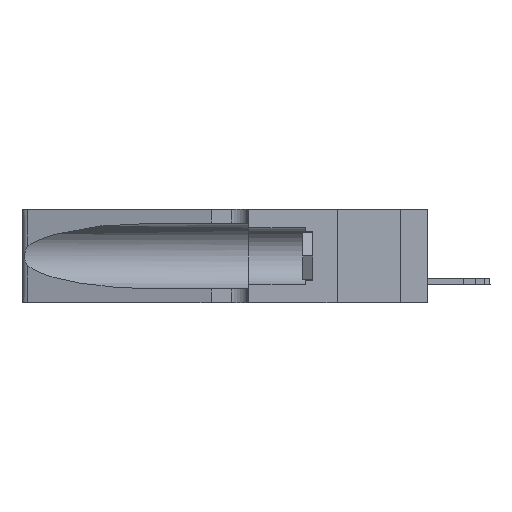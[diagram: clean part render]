
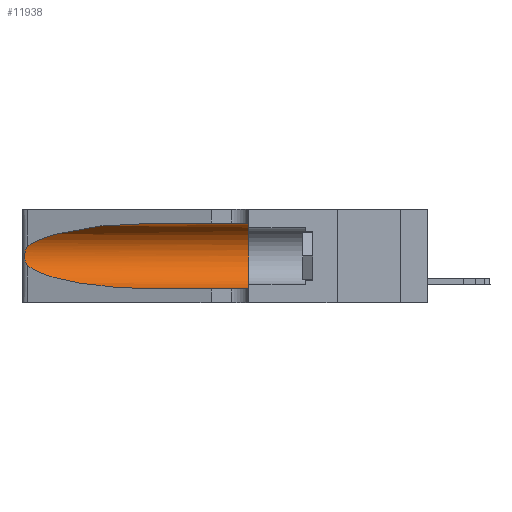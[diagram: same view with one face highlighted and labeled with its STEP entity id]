
A CAD part, left-side view. The second image highlights one B-rep face of the part: STEP entity #11938.
In plain terms, the highlighted cylindrical face has radius 3.308 mm (diameter 6.617 mm), a partial arc.
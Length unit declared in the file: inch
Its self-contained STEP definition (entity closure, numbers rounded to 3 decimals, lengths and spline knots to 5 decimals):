
#50 = CARTESIAN_POINT ( 'NONE',  ( 0.25487, 1.22718, 0.14631 ) ) ;
#316 = CARTESIAN_POINT ( 'NONE',  ( 0.25487, 1.22718, 0.14631 ) ) ;
#2418 = CARTESIAN_POINT ( 'NONE',  ( 0.25639, 1.23184, 0.21858 ) ) ;
#2800 = CARTESIAN_POINT ( 'NONE',  ( 0.26075, 1.23896, 0.178 ) ) ;
#2833 = CARTESIAN_POINT ( 'NONE',  ( 0.2373, 1.15595, 0.08982 ) ) ;
#3090 = CARTESIAN_POINT ( 'NONE',  ( 0.18966, 0.96281, 0.05475 ) ) ;
#3709 = ORIENTED_EDGE ( 'NONE', *, *, #11595, .F. ) ;
#4670 = CARTESIAN_POINT ( 'NONE',  ( 0.1305, 0.35, 0.185 ) ) ;
#4705 = VERTEX_POINT ( 'NONE', #24606 ) ;
#5203 = CARTESIAN_POINT ( 'NONE',  ( 0.25787, 1.23484, 0.2124 ) ) ;
#5291 = CARTESIAN_POINT ( 'NONE',  ( 0.1305, 1.61858, 0.05475 ) ) ;
#5942 = CARTESIAN_POINT ( 'NONE',  ( 0.25854, 1.2359, 0.20912 ) ) ;
#6542 = CARTESIAN_POINT ( 'NONE',  ( 0.25487, 1.22718, 0.22369 ) ) ;
#6719 = CARTESIAN_POINT ( 'NONE',  ( 0.1305, 0.35, 0.05475 ) ) ;
#8002 =( BOUNDED_CURVE ( )  B_SPLINE_CURVE ( 3, ( #31514, #37993, #9912, #24419 ),
 .UNSPECIFIED., .F., .T. ) 
 B_SPLINE_CURVE_WITH_KNOTS ( ( 4, 4 ),
 ( 1.5708, 2.84003 ),
 .UNSPECIFIED. ) 
 CURVE ( )  GEOMETRIC_REPRESENTATION_ITEM ( )  RATIONAL_B_SPLINE_CURVE ( ( 1., 0.87, 0.87, 1. ) ) 
 REPRESENTATION_ITEM ( '' )  );
#8210 = EDGE_CURVE ( 'NONE', #13375, #37274, #10234, .T. ) ;
#8777 = DIRECTION ( 'NONE',  ( 0., -1., 0. ) ) ;
#8936 = CARTESIAN_POINT ( 'NONE',  ( 0.26018, 1.23835, 0.19895 ) ) ;
#9583 = DIRECTION ( 'NONE',  ( 0., -1., 0. ) ) ;
#9733 = VECTOR ( 'NONE', #8777, 39.37008 ) ;
#9912 = CARTESIAN_POINT ( 'NONE',  ( 0.2373, 1.15595, 0.28018 ) ) ;
#10234 = LINE ( 'NONE', #5291, #9733 ) ;
#11203 = AXIS2_PLACEMENT_3D ( 'NONE', #16275, #13695, #31304 ) ;
#11595 = EDGE_CURVE ( 'NONE', #4705, #37274, #24460, .T. ) ;
#11734 = B_SPLINE_CURVE_WITH_KNOTS ( 'NONE', 3,
 ( #13673, #34036, #2418, #5203, #5942, #8936, #35508, #2800, #36458, #25224, #19751, #20780, #14898, #31490 ),
 .UNSPECIFIED., .F., .F.,
 ( 4, 2, 2, 2, 2, 2, 4 ),
 ( 0., 0.00027, 0.00053, 0.00107, 0.0016, 0.00187, 0.00214 ),
 .UNSPECIFIED. ) ;
#11912 = DIRECTION ( 'NONE',  ( 0., 1., 0. ) ) ;
#11938 = ADVANCED_FACE ( 'NONE', ( #29193 ), #35284, .F. ) ;
#12600 = CARTESIAN_POINT ( 'NONE',  ( 0.1305, 1.61858, 0.31525 ) ) ;
#13375 = VERTEX_POINT ( 'NONE', #24966 ) ;
#13673 = CARTESIAN_POINT ( 'NONE',  ( 0.25487, 1.22718, 0.22369 ) ) ;
#13695 = DIRECTION ( 'NONE',  ( 0., -1., 0. ) ) ;
#14027 = EDGE_CURVE ( 'NONE', #34534, #18347, #8002, .T. ) ;
#14898 = CARTESIAN_POINT ( 'NONE',  ( 0.25555, 1.22993, 0.14849 ) ) ;
#16275 = CARTESIAN_POINT ( 'NONE',  ( 0.1305, 1.61858, 0.185 ) ) ;
#18347 = VERTEX_POINT ( 'NONE', #6542 ) ;
#19069 = LINE ( 'NONE', #12600, #33106 ) ;
#19711 = AXIS2_PLACEMENT_3D ( 'NONE', #4670, #11912, #20560 ) ;
#19751 = CARTESIAN_POINT ( 'NONE',  ( 0.25789, 1.23486, 0.15765 ) ) ;
#20560 = DIRECTION ( 'NONE',  ( 0., 0., 1. ) ) ;
#20780 = CARTESIAN_POINT ( 'NONE',  ( 0.25639, 1.23186, 0.15144 ) ) ;
#23723 = CARTESIAN_POINT ( 'NONE',  ( 0.1305, 0.72297, 0.05475 ) ) ;
#24296 = EDGE_CURVE ( 'NONE', #18347, #26493, #11734, .T. ) ;
#24320 = ORIENTED_EDGE ( 'NONE', *, *, #8210, .T. ) ;
#24419 = CARTESIAN_POINT ( 'NONE',  ( 0.25487, 1.22718, 0.22369 ) ) ;
#24460 = CIRCLE ( 'NONE', #19711, 0.13025 ) ;
#24606 = CARTESIAN_POINT ( 'NONE',  ( 0.1305, 0.35, 0.31525 ) ) ;
#24935 = EDGE_LOOP ( 'NONE', ( #38352, #32174, #29657, #24320, #3709, #25769 ) ) ;
#24966 = CARTESIAN_POINT ( 'NONE',  ( 0.1305, 0.72297, 0.05475 ) ) ;
#25224 = CARTESIAN_POINT ( 'NONE',  ( 0.25856, 1.23593, 0.16098 ) ) ;
#25769 = ORIENTED_EDGE ( 'NONE', *, *, #29780, .F. ) ;
#26493 = VERTEX_POINT ( 'NONE', #316 ) ;
#26895 = CARTESIAN_POINT ( 'NONE',  ( 0.1305, 0.72297, 0.31525 ) ) ;
#29070 = EDGE_CURVE ( 'NONE', #26493, #13375, #29713, .T. ) ;
#29193 = FACE_OUTER_BOUND ( 'NONE', #24935, .T. ) ;
#29657 = ORIENTED_EDGE ( 'NONE', *, *, #29070, .T. ) ;
#29713 =( BOUNDED_CURVE ( )  B_SPLINE_CURVE ( 3, ( #50, #2833, #3090, #23723 ),
 .UNSPECIFIED., .F., .F. ) 
 B_SPLINE_CURVE_WITH_KNOTS ( ( 4, 4 ),
 ( 3.44316, 4.71239 ),
 .UNSPECIFIED. ) 
 CURVE ( )  GEOMETRIC_REPRESENTATION_ITEM ( )  RATIONAL_B_SPLINE_CURVE ( ( 1., 0.87, 0.87, 1. ) ) 
 REPRESENTATION_ITEM ( '' )  );
#29780 = EDGE_CURVE ( 'NONE', #34534, #4705, #19069, .T. ) ;
#31304 = DIRECTION ( 'NONE',  ( 0., 0., -1. ) ) ;
#31490 = CARTESIAN_POINT ( 'NONE',  ( 0.25487, 1.22718, 0.14631 ) ) ;
#31514 = CARTESIAN_POINT ( 'NONE',  ( 0.1305, 0.72297, 0.31525 ) ) ;
#32174 = ORIENTED_EDGE ( 'NONE', *, *, #24296, .T. ) ;
#33106 = VECTOR ( 'NONE', #9583, 39.37008 ) ;
#34036 = CARTESIAN_POINT ( 'NONE',  ( 0.25555, 1.22994, 0.2215 ) ) ;
#34534 = VERTEX_POINT ( 'NONE', #26895 ) ;
#35284 = CYLINDRICAL_SURFACE ( 'NONE', #11203, 0.13025 ) ;
#35508 = CARTESIAN_POINT ( 'NONE',  ( 0.26075, 1.23896, 0.19203 ) ) ;
#36458 = CARTESIAN_POINT ( 'NONE',  ( 0.26017, 1.23833, 0.17102 ) ) ;
#37274 = VERTEX_POINT ( 'NONE', #6719 ) ;
#37993 = CARTESIAN_POINT ( 'NONE',  ( 0.18966, 0.96281, 0.31525 ) ) ;
#38352 = ORIENTED_EDGE ( 'NONE', *, *, #14027, .T. ) ;
